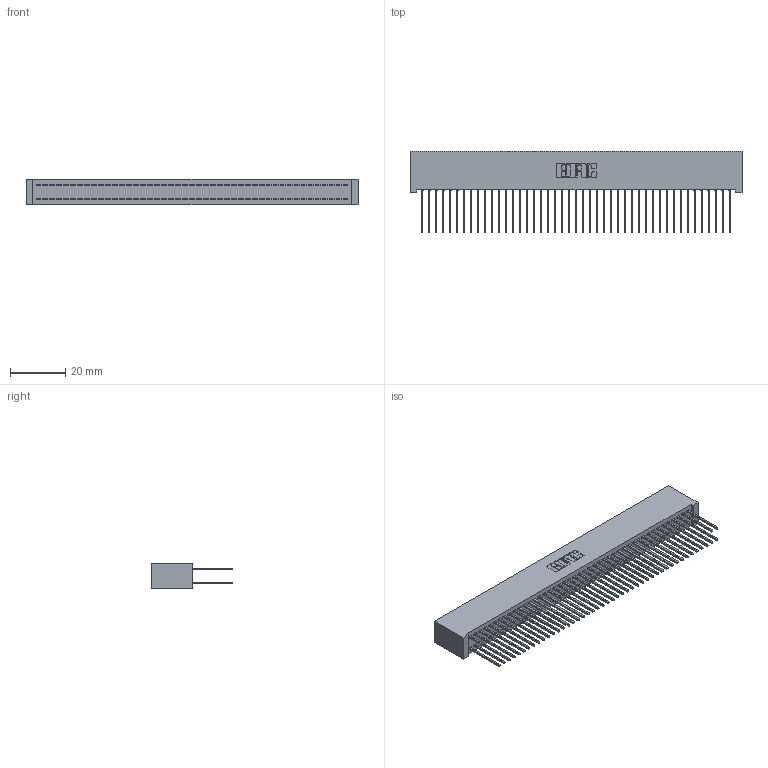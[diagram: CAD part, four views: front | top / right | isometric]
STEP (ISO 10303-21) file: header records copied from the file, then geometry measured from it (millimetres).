
FILE_DESCRIPTION (( 'STEP AP203' ), '1' );
FILE_NAME ('392-090-540-201.STEP', '2019-10-09T18:24:06', ( '' ), ( '' ), 'SwSTEP 2.0', 'SolidWorks 2016', '' );
FILE_SCHEMA (( 'CONFIG_CONTROL_DESIGN' ));
Length unit declared in the file: inch
Products named in the file (3): 342 Part_Lugless; 345-292-001_345-293-140; 392-090-540-201
Assembly tree (91 placements, depth 2):
  392-090-540-201
    342 Part_Lugless
    345-292-001_345-293-140  x90
Bounding box: 120.55 x 29.47 x 9.4 mm (x, y, z)
Volume: 11626.2 mm3; surface area: 20961.4 mm2
Topology: 91 solids, 91 shells, 4782 faces, 14225 edges, 9362 vertices
Faces by surface type: plane 3302, cylinder 1480
Entity records: 28171 total; most frequent: CARTESIAN_POINT 4662, ORIENTED_EDGE 4598, DIRECTION 3971, EDGE_CURVE 2299, VECTOR 2179, LINE 2179, VERTEX_POINT 1530, AXIS2_PLACEMENT_3D 896
